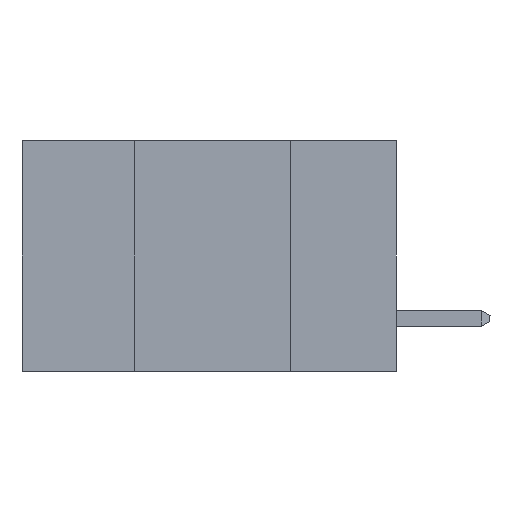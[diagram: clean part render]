
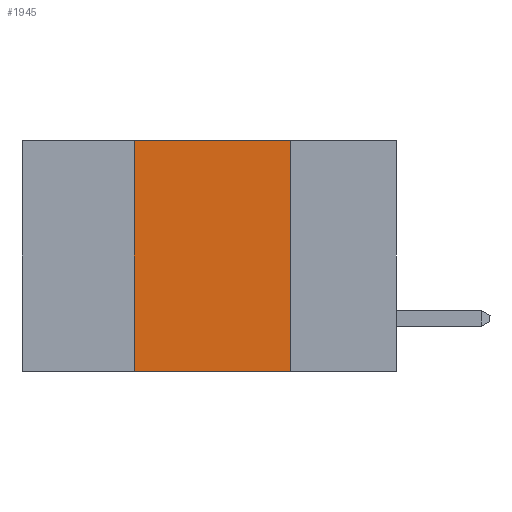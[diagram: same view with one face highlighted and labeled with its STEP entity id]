
A CAD part, left-side view. The second image highlights one B-rep face of the part: STEP entity #1945.
In plain terms, the highlighted planar face has unit normal (-1, 0, 0).
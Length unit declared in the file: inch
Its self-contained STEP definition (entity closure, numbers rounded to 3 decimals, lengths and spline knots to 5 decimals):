
#140 = LINE ( 'NONE', #4852, #2937 ) ;
#204 = VERTEX_POINT ( 'NONE', #5232 ) ;
#987 = LINE ( 'NONE', #11963, #5847 ) ;
#1588 = CARTESIAN_POINT ( 'NONE',  ( 0., 0.42, -0.37 ) ) ;
#1828 = ORIENTED_EDGE ( 'NONE', *, *, #7935, .F. ) ;
#1945 = ADVANCED_FACE ( 'NONE', ( #5268 ), #7528, .F. ) ;
#2034 = ORIENTED_EDGE ( 'NONE', *, *, #8597, .F. ) ;
#2167 = ORIENTED_EDGE ( 'NONE', *, *, #2305, .F. ) ;
#2181 = ORIENTED_EDGE ( 'NONE', *, *, #2252, .T. ) ;
#2252 = EDGE_CURVE ( 'NONE', #12585, #4316, #987, .T. ) ;
#2305 = EDGE_CURVE ( 'NONE', #12585, #204, #12457, .T. ) ;
#2937 = VECTOR ( 'NONE', #11494, 39.37008 ) ;
#3845 = CARTESIAN_POINT ( 'NONE',  ( 0., 0.17, -0.37 ) ) ;
#4090 = CARTESIAN_POINT ( 'NONE',  ( 0., 0.17, -0.37 ) ) ;
#4316 = VERTEX_POINT ( 'NONE', #3845 ) ;
#4661 = VECTOR ( 'NONE', #10149, 39.37008 ) ;
#4755 = VECTOR ( 'NONE', #10764, 39.37008 ) ;
#4852 = CARTESIAN_POINT ( 'NONE',  ( 0., 0.6, 0. ) ) ;
#5232 = CARTESIAN_POINT ( 'NONE',  ( 0., 0.42, 0. ) ) ;
#5268 = FACE_OUTER_BOUND ( 'NONE', #9181, .T. ) ;
#5584 = AXIS2_PLACEMENT_3D ( 'NONE', #7655, #8171, #7492 ) ;
#5847 = VECTOR ( 'NONE', #11975, 39.37008 ) ;
#6179 = CARTESIAN_POINT ( 'NONE',  ( 0., 0.17, 0. ) ) ;
#7492 = DIRECTION ( 'NONE',  ( 0., 0., -1. ) ) ;
#7528 = PLANE ( 'NONE',  #5584 ) ;
#7655 = CARTESIAN_POINT ( 'NONE',  ( 0., 0.6, 0. ) ) ;
#7928 = LINE ( 'NONE', #4090, #4755 ) ;
#7935 = EDGE_CURVE ( 'NONE', #11189, #4316, #7928, .T. ) ;
#8171 = DIRECTION ( 'NONE',  ( 1., 0., 0. ) ) ;
#8201 = CARTESIAN_POINT ( 'NONE',  ( 0., 0.42, -0.37 ) ) ;
#8597 = EDGE_CURVE ( 'NONE', #204, #11189, #140, .T. ) ;
#9181 = EDGE_LOOP ( 'NONE', ( #1828, #2034, #2167, #2181 ) ) ;
#10149 = DIRECTION ( 'NONE',  ( 0., 0., 1. ) ) ;
#10764 = DIRECTION ( 'NONE',  ( 0., 0., -1. ) ) ;
#11189 = VERTEX_POINT ( 'NONE', #6179 ) ;
#11494 = DIRECTION ( 'NONE',  ( 0., -1., 0. ) ) ;
#11963 = CARTESIAN_POINT ( 'NONE',  ( 0., 0.6, -0.37 ) ) ;
#11975 = DIRECTION ( 'NONE',  ( 0., -1., 0. ) ) ;
#12457 = LINE ( 'NONE', #1588, #4661 ) ;
#12585 = VERTEX_POINT ( 'NONE', #8201 ) ;
